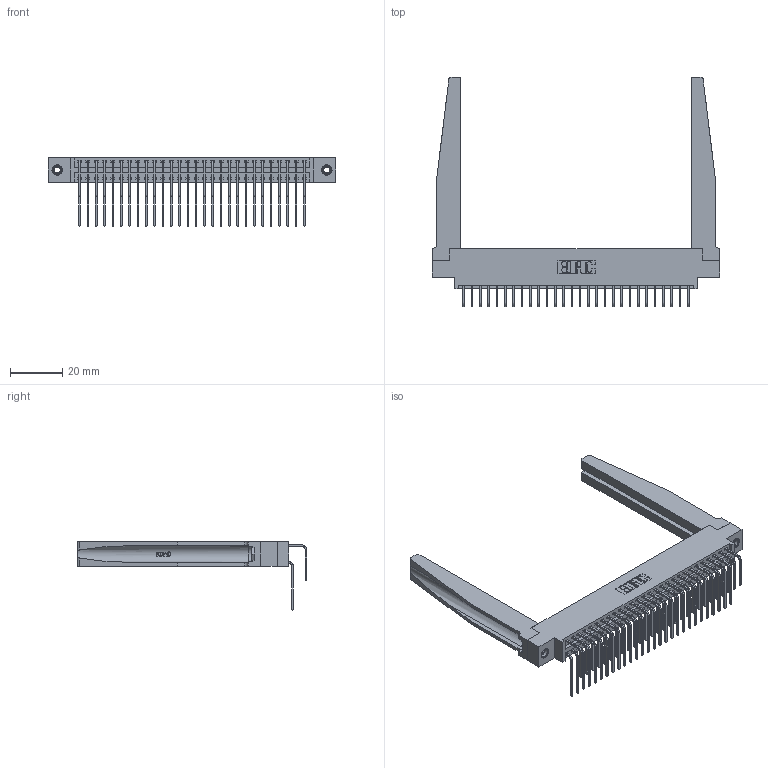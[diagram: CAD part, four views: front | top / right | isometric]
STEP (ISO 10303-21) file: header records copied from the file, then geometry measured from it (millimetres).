
FILE_DESCRIPTION (( 'STEP AP203' ), '1' );
FILE_NAME ('396-056-558-878.STEP', '2019-11-03T09:19:06', ( '' ), ( '' ), 'SwSTEP 2.0', 'SolidWorks 2016', '' );
FILE_SCHEMA (( 'CONFIG_CONTROL_DESIGN' ));
Length unit declared in the file: inch
Products named in the file (6): 346 Part_0.170 Offset - 0.156 Dia-TH; 345-292-001_558 Tail - 2; 345-292-001_558 559 Tail - 1; 346-220-078_345-220-078; 345-250-001_345-250-001-102; 396-056-558-878
Assembly tree (61 placements, depth 2):
  396-056-558-878
    346 Part_0.170 Offset - 0.156 Dia-TH
    345-292-001_558 559 Tail - 1  x28
    345-292-001_558 Tail - 2  x28
    346-220-078_345-220-078  x2
    345-250-001_345-250-001-102  x2
Bounding box: 109.47 x 87.44 x 26.16 mm (x, y, z)
Volume: 17643.6 mm3; surface area: 22802.5 mm2
Topology: 61 solids, 61 shells, 3384 faces, 9965 edges, 6558 vertices
Faces by surface type: plane 2294, cylinder 1038, bspline 36, cone 12, torus 4
Entity records: 26822 total; most frequent: CARTESIAN_POINT 5430, ORIENTED_EDGE 4202, DIRECTION 3795, EDGE_CURVE 2101, VECTOR 1723, LINE 1723, VERTEX_POINT 1392, AXIS2_PLACEMENT_3D 1036
